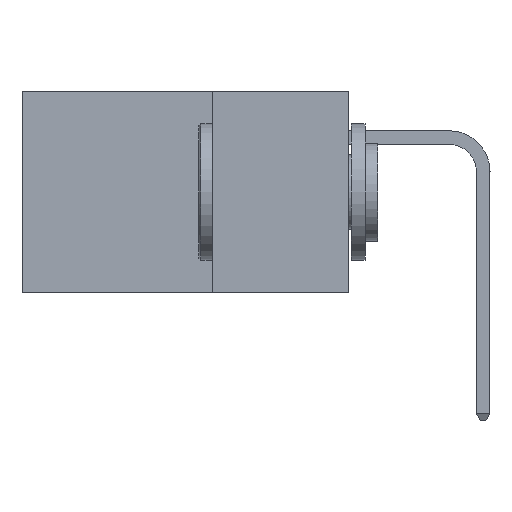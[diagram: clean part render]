
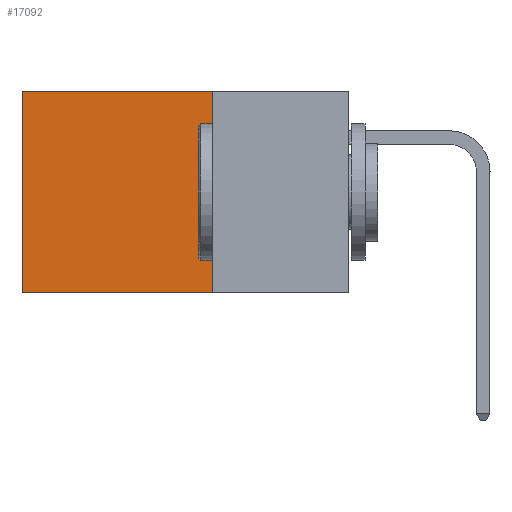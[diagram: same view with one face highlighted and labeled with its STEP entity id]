
A CAD part, left-side view. The second image highlights one B-rep face of the part: STEP entity #17092.
In plain terms, the highlighted planar face has unit normal (-1, 0, 0).
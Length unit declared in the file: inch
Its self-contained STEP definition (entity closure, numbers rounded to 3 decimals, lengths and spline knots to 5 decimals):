
#247 = ORIENTED_EDGE ( 'NONE', *, *, #4887, .F. ) ;
#1347 = DIRECTION ( 'NONE',  ( 0., 0., -1. ) ) ;
#2649 = EDGE_CURVE ( 'NONE', #18088, #16360, #14910, .T. ) ;
#3229 = VECTOR ( 'NONE', #16165, 39.37008 ) ;
#3300 = CARTESIAN_POINT ( 'NONE',  ( 0.2875, 0.25, -0.37 ) ) ;
#3336 = EDGE_CURVE ( 'NONE', #4886, #18548, #11324, .T. ) ;
#3523 = VECTOR ( 'NONE', #5286, 39.37008 ) ;
#3707 = LINE ( 'NONE', #16239, #3229 ) ;
#4328 = FACE_OUTER_BOUND ( 'NONE', #11717, .T. ) ;
#4816 = ORIENTED_EDGE ( 'NONE', *, *, #3336, .T. ) ;
#4886 = VERTEX_POINT ( 'NONE', #16286 ) ;
#4887 = EDGE_CURVE ( 'NONE', #4886, #18088, #3707, .T. ) ;
#5286 = DIRECTION ( 'NONE',  ( 0., 1., 0. ) ) ;
#6016 = CARTESIAN_POINT ( 'NONE',  ( 0.2875, 0.25, 0. ) ) ;
#6112 = LINE ( 'NONE', #6208, #6565 ) ;
#6208 = CARTESIAN_POINT ( 'NONE',  ( 0.2875, 0.6, 0. ) ) ;
#6275 = DIRECTION ( 'NONE',  ( 0., 0., -1. ) ) ;
#6328 = ORIENTED_EDGE ( 'NONE', *, *, #11393, .T. ) ;
#6565 = VECTOR ( 'NONE', #6275, 39.37008 ) ;
#10248 = DIRECTION ( 'NONE',  ( 1., 0., 0. ) ) ;
#11124 = VECTOR ( 'NONE', #13639, 39.37008 ) ;
#11324 = LINE ( 'NONE', #6016, #3523 ) ;
#11393 = EDGE_CURVE ( 'NONE', #18548, #16360, #6112, .T. ) ;
#11717 = EDGE_LOOP ( 'NONE', ( #6328, #13514, #247, #4816 ) ) ;
#13146 = PLANE ( 'NONE',  #18402 ) ;
#13514 = ORIENTED_EDGE ( 'NONE', *, *, #2649, .F. ) ;
#13639 = DIRECTION ( 'NONE',  ( 0., 1., 0. ) ) ;
#13815 = CARTESIAN_POINT ( 'NONE',  ( 0.2875, 0.25, -0.37 ) ) ;
#14910 = LINE ( 'NONE', #13815, #11124 ) ;
#16165 = DIRECTION ( 'NONE',  ( 0., 0., -1. ) ) ;
#16239 = CARTESIAN_POINT ( 'NONE',  ( 0.2875, 0.25, 0. ) ) ;
#16286 = CARTESIAN_POINT ( 'NONE',  ( 0.2875, 0.25, 0. ) ) ;
#16360 = VERTEX_POINT ( 'NONE', #17937 ) ;
#17092 = ADVANCED_FACE ( 'NONE', ( #4328 ), #13146, .F. ) ;
#17937 = CARTESIAN_POINT ( 'NONE',  ( 0.2875, 0.6, -0.37 ) ) ;
#18088 = VERTEX_POINT ( 'NONE', #3300 ) ;
#18402 = AXIS2_PLACEMENT_3D ( 'NONE', #18550, #10248, #1347 ) ;
#18548 = VERTEX_POINT ( 'NONE', #18622 ) ;
#18550 = CARTESIAN_POINT ( 'NONE',  ( 0.2875, 0.25, 0. ) ) ;
#18622 = CARTESIAN_POINT ( 'NONE',  ( 0.2875, 0.6, 0. ) ) ;
